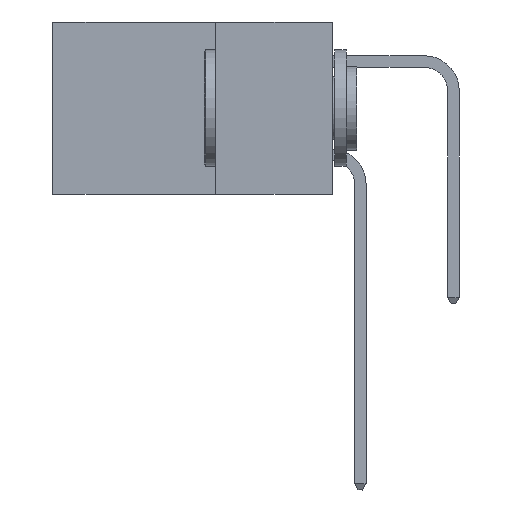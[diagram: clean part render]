
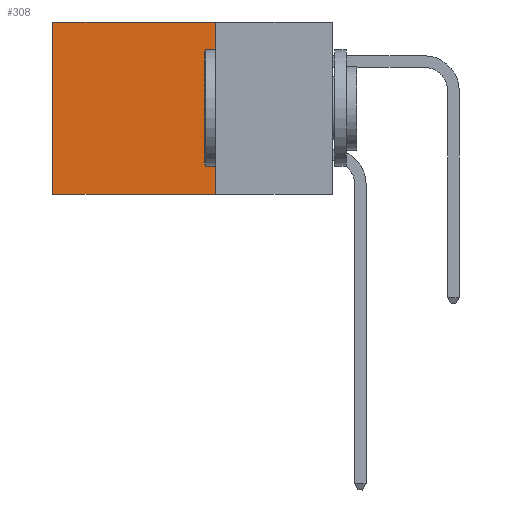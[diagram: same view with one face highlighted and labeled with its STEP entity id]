
A CAD part, left-side view. The second image highlights one B-rep face of the part: STEP entity #308.
In plain terms, the highlighted planar face has unit normal (-1, 0, 0).
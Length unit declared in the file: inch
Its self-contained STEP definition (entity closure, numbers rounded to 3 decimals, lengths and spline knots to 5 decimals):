
#308 = ADVANCED_FACE ( 'NONE', ( #822 ), #20973, .F. ) ;
#529 = DIRECTION ( 'NONE',  ( 0., 0., -1. ) ) ;
#666 = ORIENTED_EDGE ( 'NONE', *, *, #18659, .F. ) ;
#822 = FACE_OUTER_BOUND ( 'NONE', #15305, .T. ) ;
#836 = EDGE_CURVE ( 'NONE', #22809, #9630, #4098, .T. ) ;
#2182 = CARTESIAN_POINT ( 'NONE',  ( 0.2615, 0.6, 0. ) ) ;
#2642 = EDGE_CURVE ( 'NONE', #3899, #22809, #10533, .T. ) ;
#2936 = EDGE_CURVE ( 'NONE', #9892, #9630, #9658, .T. ) ;
#3899 = VERTEX_POINT ( 'NONE', #7185 ) ;
#4098 = LINE ( 'NONE', #8145, #8528 ) ;
#5519 = DIRECTION ( 'NONE',  ( 0., 1., 0. ) ) ;
#6074 = CARTESIAN_POINT ( 'NONE',  ( 0.2615, 0.6, -0.37 ) ) ;
#6302 = ORIENTED_EDGE ( 'NONE', *, *, #2936, .F. ) ;
#7185 = CARTESIAN_POINT ( 'NONE',  ( 0.2615, 0.25, 0. ) ) ;
#8145 = CARTESIAN_POINT ( 'NONE',  ( 0.2615, 0.6, -0.37 ) ) ;
#8528 = VECTOR ( 'NONE', #10056, 39.37008 ) ;
#8744 = CARTESIAN_POINT ( 'NONE',  ( 0.2615, 0.25, 0. ) ) ;
#9630 = VERTEX_POINT ( 'NONE', #6074 ) ;
#9658 = LINE ( 'NONE', #19349, #23382 ) ;
#9892 = VERTEX_POINT ( 'NONE', #16071 ) ;
#10056 = DIRECTION ( 'NONE',  ( 0., 0., -1. ) ) ;
#10533 = LINE ( 'NONE', #8744, #19907 ) ;
#15015 = ORIENTED_EDGE ( 'NONE', *, *, #2642, .T. ) ;
#15305 = EDGE_LOOP ( 'NONE', ( #23679, #6302, #666, #15015 ) ) ;
#16071 = CARTESIAN_POINT ( 'NONE',  ( 0.2615, 0.25, -0.37 ) ) ;
#17471 = DIRECTION ( 'NONE',  ( 0., 0., -1. ) ) ;
#18631 = VECTOR ( 'NONE', #529, 39.37008 ) ;
#18659 = EDGE_CURVE ( 'NONE', #3899, #9892, #23567, .T. ) ;
#19349 = CARTESIAN_POINT ( 'NONE',  ( 0.2615, 0.25, -0.37 ) ) ;
#19381 = DIRECTION ( 'NONE',  ( 0., 1., 0. ) ) ;
#19907 = VECTOR ( 'NONE', #5519, 39.37008 ) ;
#20892 = DIRECTION ( 'NONE',  ( 1., 0., 0. ) ) ;
#20973 = PLANE ( 'NONE',  #21850 ) ;
#21000 = CARTESIAN_POINT ( 'NONE',  ( 0.2615, 0.25, -0.37 ) ) ;
#21850 = AXIS2_PLACEMENT_3D ( 'NONE', #21000, #20892, #17471 ) ;
#22809 = VERTEX_POINT ( 'NONE', #2182 ) ;
#23060 = CARTESIAN_POINT ( 'NONE',  ( 0.2615, 0.25, -0.37 ) ) ;
#23382 = VECTOR ( 'NONE', #19381, 39.37008 ) ;
#23567 = LINE ( 'NONE', #23060, #18631 ) ;
#23679 = ORIENTED_EDGE ( 'NONE', *, *, #836, .T. ) ;
